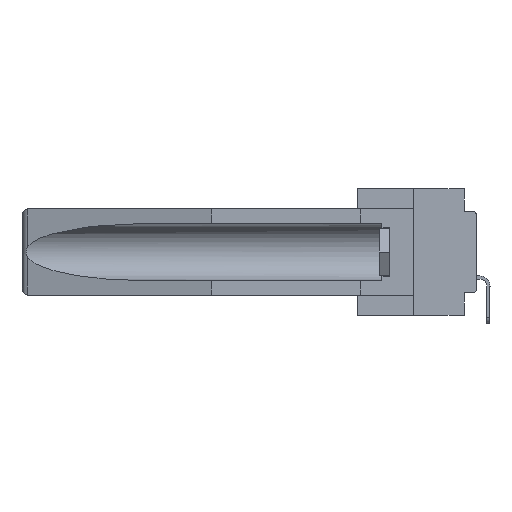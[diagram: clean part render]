
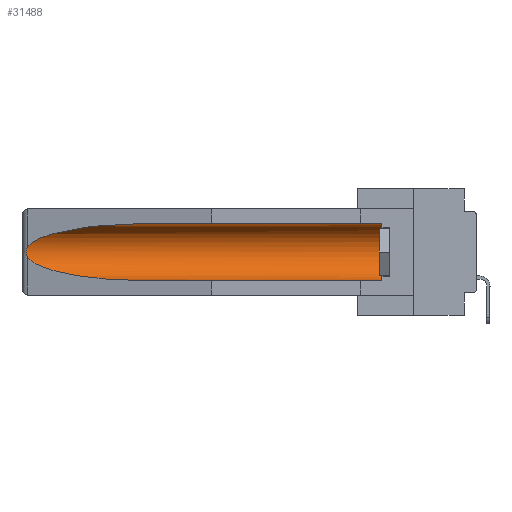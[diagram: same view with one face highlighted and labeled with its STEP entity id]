
A CAD part, left-side view. The second image highlights one B-rep face of the part: STEP entity #31488.
In plain terms, the highlighted cylindrical face has radius 2.857 mm (diameter 5.715 mm), a partial arc.
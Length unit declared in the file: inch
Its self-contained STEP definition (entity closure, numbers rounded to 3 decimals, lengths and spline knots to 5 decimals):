
#121 = VERTEX_POINT ( 'NONE', #30777 ) ;
#958 = ORIENTED_EDGE ( 'NONE', *, *, #9943, .T. ) ;
#1123 = EDGE_LOOP ( 'NONE', ( #15102, #22982, #16220, #25425, #27048, #958 ) ) ;
#1244 = AXIS2_PLACEMENT_3D ( 'NONE', #32829, #4652, #21751 ) ;
#1837 = CARTESIAN_POINT ( 'NONE',  ( 0.26537, 1.52718, -0.19328 ) ) ;
#2137 = CARTESIAN_POINT ( 'NONE',  ( 0.25451, 1.48313, -0.24835 ) ) ;
#2266 = DIRECTION ( 'NONE',  ( 0., 0., 1. ) ) ;
#2924 = VECTOR ( 'NONE', #10025, 39.37008 ) ;
#4652 = DIRECTION ( 'NONE',  ( 0., 1., 0. ) ) ;
#4852 = CARTESIAN_POINT ( 'NONE',  ( 0.21114, 1.30732, -0.059 ) ) ;
#5504 = EDGE_CURVE ( 'NONE', #121, #25446, #20073, .T. ) ;
#6160 = VERTEX_POINT ( 'NONE', #13430 ) ;
#6899 = CARTESIAN_POINT ( 'NONE',  ( 0.25451, 1.48313, -0.09465 ) ) ;
#7377 = CARTESIAN_POINT ( 'NONE',  ( 0.26597, 1.52961, -0.15275 ) ) ;
#8775 = EDGE_CURVE ( 'NONE', #25446, #11989, #20864, .T. ) ;
#9940 = CARTESIAN_POINT ( 'NONE',  ( 0.155, 0.126, -0.059 ) ) ;
#9943 = EDGE_CURVE ( 'NONE', #21887, #6160, #32021, .T. ) ;
#10025 = DIRECTION ( 'NONE',  ( 0., 1., 0. ) ) ;
#11989 = VERTEX_POINT ( 'NONE', #14138 ) ;
#13430 = CARTESIAN_POINT ( 'NONE',  ( 0.155, 1.07973, -0.059 ) ) ;
#13580 =( BOUNDED_CURVE ( )  B_SPLINE_CURVE ( 3, ( #27112, #4852, #6899, #24356 ),
 .UNSPECIFIED., .F., .F. ) 
 B_SPLINE_CURVE_WITH_KNOTS ( ( 4, 4 ),
 ( 4.71239, 6.08839 ),
 .UNSPECIFIED. ) 
 CURVE ( )  GEOMETRIC_REPRESENTATION_ITEM ( )  RATIONAL_B_SPLINE_CURVE ( ( 1., 0.848, 0.848, 1. ) ) 
 REPRESENTATION_ITEM ( '' )  );
#14138 = CARTESIAN_POINT ( 'NONE',  ( 0.155, 1.07973, -0.284 ) ) ;
#15102 = ORIENTED_EDGE ( 'NONE', *, *, #17026, .T. ) ;
#15826 = DIRECTION ( 'NONE',  ( 0., 1., 0. ) ) ;
#15843 = CARTESIAN_POINT ( 'NONE',  ( 0.155, 0.126, -0.284 ) ) ;
#15857 = CARTESIAN_POINT ( 'NONE',  ( 0.2675, 1.53308, -0.16763 ) ) ;
#16220 = ORIENTED_EDGE ( 'NONE', *, *, #8775, .T. ) ;
#16311 = CARTESIAN_POINT ( 'NONE',  ( 0.155, -0.30754, -0.284 ) ) ;
#17026 = EDGE_CURVE ( 'NONE', #6160, #121, #13580, .T. ) ;
#19211 = CARTESIAN_POINT ( 'NONE',  ( 0.155, 0.126, -0.1715 ) ) ;
#20073 = B_SPLINE_CURVE_WITH_KNOTS ( 'NONE', 3,
 ( #30018, #7377, #26688, #23928, #15857, #35180, #29456, #32055, #23557, #1837 ),
 .UNSPECIFIED., .F., .F.,
 ( 4, 2, 2, 2, 4 ),
 ( 0., 0.00029, 0.00058, 0.00087, 0.00117 ),
 .UNSPECIFIED. ) ;
#20563 = VERTEX_POINT ( 'NONE', #15843 ) ;
#20780 = CARTESIAN_POINT ( 'NONE',  ( 0.155, -0.30754, -0.059 ) ) ;
#20864 =( BOUNDED_CURVE ( )  B_SPLINE_CURVE ( 3, ( #27543, #2137, #32707, #26798 ),
 .UNSPECIFIED., .F., .F. ) 
 B_SPLINE_CURVE_WITH_KNOTS ( ( 4, 4 ),
 ( 0.1948, 1.5708 ),
 .UNSPECIFIED. ) 
 CURVE ( )  GEOMETRIC_REPRESENTATION_ITEM ( )  RATIONAL_B_SPLINE_CURVE ( ( 1., 0.848, 0.848, 1. ) ) 
 REPRESENTATION_ITEM ( '' )  );
#21751 = DIRECTION ( 'NONE',  ( 0., 0., 1. ) ) ;
#21758 = DIRECTION ( 'NONE',  ( 0., -1., 0. ) ) ;
#21887 = VERTEX_POINT ( 'NONE', #9940 ) ;
#22982 = ORIENTED_EDGE ( 'NONE', *, *, #5504, .T. ) ;
#23557 = CARTESIAN_POINT ( 'NONE',  ( 0.26597, 1.5296, -0.19026 ) ) ;
#23928 = CARTESIAN_POINT ( 'NONE',  ( 0.2673, 1.5327, -0.16383 ) ) ;
#24140 = CYLINDRICAL_SURFACE ( 'NONE', #1244, 0.1125 ) ;
#24356 = CARTESIAN_POINT ( 'NONE',  ( 0.26537, 1.52718, -0.14972 ) ) ;
#24563 = EDGE_CURVE ( 'NONE', #20563, #21887, #27996, .T. ) ;
#25349 = CARTESIAN_POINT ( 'NONE',  ( 0.26537, 1.52718, -0.19328 ) ) ;
#25425 = ORIENTED_EDGE ( 'NONE', *, *, #29816, .F. ) ;
#25446 = VERTEX_POINT ( 'NONE', #25349 ) ;
#26688 = CARTESIAN_POINT ( 'NONE',  ( 0.26654, 1.53092, -0.15636 ) ) ;
#26798 = CARTESIAN_POINT ( 'NONE',  ( 0.155, 1.07973, -0.284 ) ) ;
#27048 = ORIENTED_EDGE ( 'NONE', *, *, #24563, .T. ) ;
#27112 = CARTESIAN_POINT ( 'NONE',  ( 0.155, 1.07973, -0.059 ) ) ;
#27543 = CARTESIAN_POINT ( 'NONE',  ( 0.26537, 1.52718, -0.19328 ) ) ;
#27996 = CIRCLE ( 'NONE', #29174, 0.1125 ) ;
#29174 = AXIS2_PLACEMENT_3D ( 'NONE', #19211, #21758, #2266 ) ;
#29456 = CARTESIAN_POINT ( 'NONE',  ( 0.2673, 1.53269, -0.17917 ) ) ;
#29816 = EDGE_CURVE ( 'NONE', #20563, #11989, #32478, .T. ) ;
#30018 = CARTESIAN_POINT ( 'NONE',  ( 0.26537, 1.52718, -0.14972 ) ) ;
#30777 = CARTESIAN_POINT ( 'NONE',  ( 0.26537, 1.52718, -0.14972 ) ) ;
#31488 = ADVANCED_FACE ( 'NONE', ( #33000 ), #24140, .F. ) ;
#32021 = LINE ( 'NONE', #20780, #34166 ) ;
#32055 = CARTESIAN_POINT ( 'NONE',  ( 0.26655, 1.53094, -0.18657 ) ) ;
#32478 = LINE ( 'NONE', #16311, #2924 ) ;
#32707 = CARTESIAN_POINT ( 'NONE',  ( 0.21114, 1.30732, -0.284 ) ) ;
#32829 = CARTESIAN_POINT ( 'NONE',  ( 0.155, -0.30754, -0.1715 ) ) ;
#33000 = FACE_OUTER_BOUND ( 'NONE', #1123, .T. ) ;
#34166 = VECTOR ( 'NONE', #15826, 39.37008 ) ;
#35180 = CARTESIAN_POINT ( 'NONE',  ( 0.2675, 1.53308, -0.17534 ) ) ;
